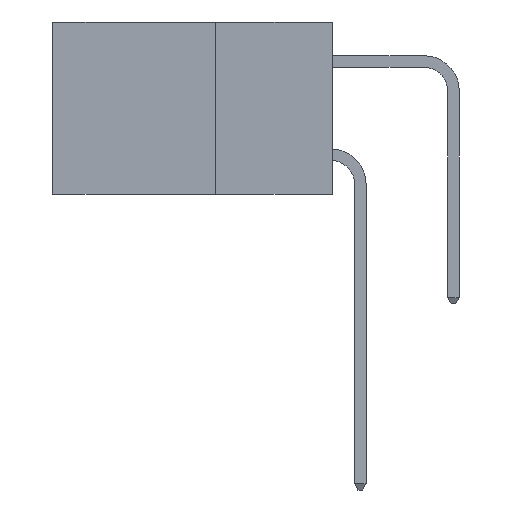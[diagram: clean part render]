
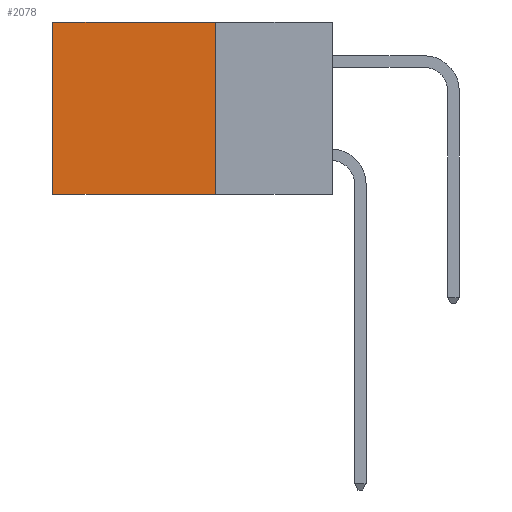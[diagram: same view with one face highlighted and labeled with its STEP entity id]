
A CAD part, left-side view. The second image highlights one B-rep face of the part: STEP entity #2078.
In plain terms, the highlighted planar face has unit normal (-1, 0, 0).
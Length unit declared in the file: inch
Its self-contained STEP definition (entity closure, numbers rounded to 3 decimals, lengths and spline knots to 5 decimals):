
#68 = CARTESIAN_POINT ( 'NONE',  ( 0.2615, 0.6, 0. ) ) ;
#498 = LINE ( 'NONE', #4295, #3083 ) ;
#1158 = CARTESIAN_POINT ( 'NONE',  ( 0.2615, 0.25, -0.37 ) ) ;
#1584 = EDGE_CURVE ( 'NONE', #4094, #11455, #7709, .T. ) ;
#1689 = LINE ( 'NONE', #9120, #11353 ) ;
#2078 = ADVANCED_FACE ( 'NONE', ( #3162 ), #14815, .F. ) ;
#3083 = VECTOR ( 'NONE', #4276, 39.37008 ) ;
#3162 = FACE_OUTER_BOUND ( 'NONE', #11770, .T. ) ;
#3569 = VECTOR ( 'NONE', #14097, 39.37008 ) ;
#3852 = EDGE_CURVE ( 'NONE', #14649, #14251, #1689, .T. ) ;
#3893 = EDGE_CURVE ( 'NONE', #4094, #14649, #7635, .T. ) ;
#4094 = VERTEX_POINT ( 'NONE', #7397 ) ;
#4276 = DIRECTION ( 'NONE',  ( 0., 1., 0. ) ) ;
#4295 = CARTESIAN_POINT ( 'NONE',  ( 0.2615, 0.25, -0.37 ) ) ;
#4357 = DIRECTION ( 'NONE',  ( 0., 1., 0. ) ) ;
#4462 = EDGE_CURVE ( 'NONE', #11455, #14251, #498, .T. ) ;
#5517 = ORIENTED_EDGE ( 'NONE', *, *, #3852, .T. ) ;
#7397 = CARTESIAN_POINT ( 'NONE',  ( 0.2615, 0.25, 0. ) ) ;
#7635 = LINE ( 'NONE', #8804, #14231 ) ;
#7709 = LINE ( 'NONE', #14143, #3569 ) ;
#7868 = CARTESIAN_POINT ( 'NONE',  ( 0.2615, 0.6, -0.37 ) ) ;
#7902 = AXIS2_PLACEMENT_3D ( 'NONE', #14970, #15221, #15115 ) ;
#8804 = CARTESIAN_POINT ( 'NONE',  ( 0.2615, 0.25, 0. ) ) ;
#8980 = ORIENTED_EDGE ( 'NONE', *, *, #4462, .F. ) ;
#9116 = DIRECTION ( 'NONE',  ( 0., 0., -1. ) ) ;
#9120 = CARTESIAN_POINT ( 'NONE',  ( 0.2615, 0.6, -0.37 ) ) ;
#11353 = VECTOR ( 'NONE', #9116, 39.37008 ) ;
#11455 = VERTEX_POINT ( 'NONE', #1158 ) ;
#11770 = EDGE_LOOP ( 'NONE', ( #5517, #8980, #12087, #13985 ) ) ;
#12087 = ORIENTED_EDGE ( 'NONE', *, *, #1584, .F. ) ;
#13985 = ORIENTED_EDGE ( 'NONE', *, *, #3893, .T. ) ;
#14097 = DIRECTION ( 'NONE',  ( 0., 0., -1. ) ) ;
#14143 = CARTESIAN_POINT ( 'NONE',  ( 0.2615, 0.25, -0.37 ) ) ;
#14231 = VECTOR ( 'NONE', #4357, 39.37008 ) ;
#14251 = VERTEX_POINT ( 'NONE', #7868 ) ;
#14649 = VERTEX_POINT ( 'NONE', #68 ) ;
#14815 = PLANE ( 'NONE',  #7902 ) ;
#14970 = CARTESIAN_POINT ( 'NONE',  ( 0.2615, 0.25, -0.37 ) ) ;
#15115 = DIRECTION ( 'NONE',  ( 0., 0., -1. ) ) ;
#15221 = DIRECTION ( 'NONE',  ( 1., 0., 0. ) ) ;
